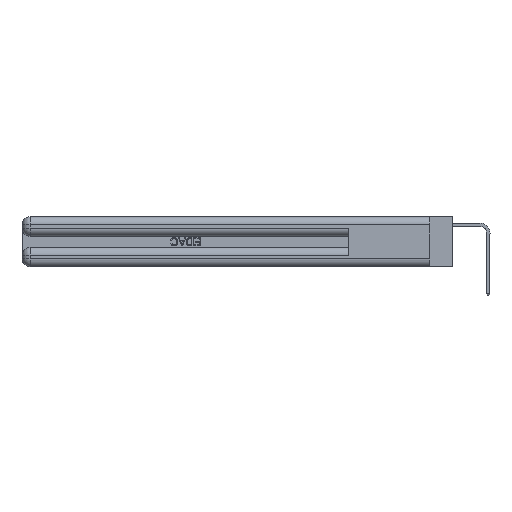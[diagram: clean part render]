
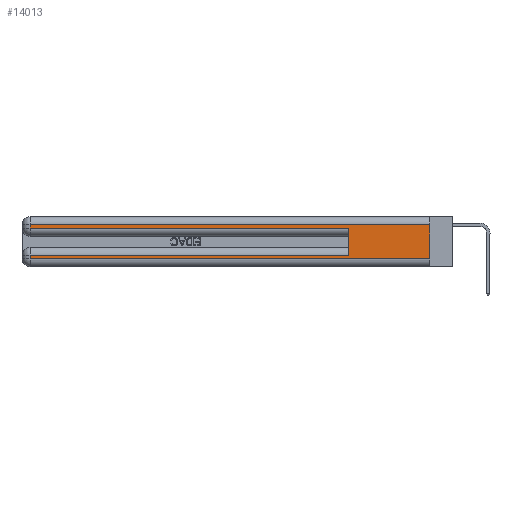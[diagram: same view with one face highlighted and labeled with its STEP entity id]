
A CAD part, left-side view. The second image highlights one B-rep face of the part: STEP entity #14013.
In plain terms, the highlighted planar face has unit normal (-1, 0, 0).
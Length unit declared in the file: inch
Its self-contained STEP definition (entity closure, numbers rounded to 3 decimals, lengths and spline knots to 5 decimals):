
#385 = VERTEX_POINT ( 'NONE', #19764 ) ;
#871 = EDGE_LOOP ( 'NONE', ( #8453, #5865, #25730, #26831, #24875, #24241, #18134, #9044 ) ) ;
#1074 = VERTEX_POINT ( 'NONE', #26707 ) ;
#1160 = VECTOR ( 'NONE', #17852, 39.37008 ) ;
#1462 = EDGE_CURVE ( 'NONE', #13988, #29570, #9830, .T. ) ;
#2735 = CARTESIAN_POINT ( 'NONE',  ( 0., 0.6, 0.145 ) ) ;
#3069 = VERTEX_POINT ( 'NONE', #13011 ) ;
#3277 = LINE ( 'NONE', #25673, #24214 ) ;
#4062 = CARTESIAN_POINT ( 'NONE',  ( 0., 2.94, 0.37 ) ) ;
#4281 = VERTEX_POINT ( 'NONE', #10620 ) ;
#5865 = ORIENTED_EDGE ( 'NONE', *, *, #6195, .T. ) ;
#6195 = EDGE_CURVE ( 'NONE', #385, #13988, #25769, .T. ) ;
#6279 = PLANE ( 'NONE',  #23796 ) ;
#7234 = DIRECTION ( 'NONE',  ( 0., 1., 0. ) ) ;
#7324 = DIRECTION ( 'NONE',  ( 0., 0., -1. ) ) ;
#7398 = LINE ( 'NONE', #4062, #1160 ) ;
#7439 = DIRECTION ( 'NONE',  ( 0., 0., 1. ) ) ;
#8453 = ORIENTED_EDGE ( 'NONE', *, *, #9283, .F. ) ;
#8616 = DIRECTION ( 'NONE',  ( 1., 0., 0. ) ) ;
#9044 = ORIENTED_EDGE ( 'NONE', *, *, #14496, .T. ) ;
#9283 = EDGE_CURVE ( 'NONE', #385, #25598, #14305, .T. ) ;
#9304 = LINE ( 'NONE', #13502, #20810 ) ;
#9428 = VECTOR ( 'NONE', #21747, 39.37008 ) ;
#9830 = LINE ( 'NONE', #23413, #22073 ) ;
#10157 = CARTESIAN_POINT ( 'NONE',  ( 0., 0., 0.31 ) ) ;
#10620 = CARTESIAN_POINT ( 'NONE',  ( 0., 2.94, 0.06 ) ) ;
#12469 = DIRECTION ( 'NONE',  ( 0., 1., 0. ) ) ;
#13011 = CARTESIAN_POINT ( 'NONE',  ( 0., 0.6, 0.285 ) ) ;
#13502 = CARTESIAN_POINT ( 'NONE',  ( 0., 0., 0.285 ) ) ;
#13506 = VECTOR ( 'NONE', #12469, 39.37008 ) ;
#13988 = VERTEX_POINT ( 'NONE', #22283 ) ;
#14013 = ADVANCED_FACE ( 'NONE', ( #28584 ), #6279, .F. ) ;
#14305 = LINE ( 'NONE', #24133, #25836 ) ;
#14496 = EDGE_CURVE ( 'NONE', #4281, #25598, #27802, .T. ) ;
#14603 = CARTESIAN_POINT ( 'NONE',  ( 0., 0.6, 0.085 ) ) ;
#14954 = VERTEX_POINT ( 'NONE', #14603 ) ;
#14994 = DIRECTION ( 'NONE',  ( 0., 0., -1. ) ) ;
#15809 = DIRECTION ( 'NONE',  ( 0., -1., 0. ) ) ;
#17852 = DIRECTION ( 'NONE',  ( 0., 0., -1. ) ) ;
#18134 = ORIENTED_EDGE ( 'NONE', *, *, #19094, .T. ) ;
#18166 = CARTESIAN_POINT ( 'NONE',  ( 0., 0., 0.06 ) ) ;
#19094 = EDGE_CURVE ( 'NONE', #1074, #4281, #7398, .T. ) ;
#19764 = CARTESIAN_POINT ( 'NONE',  ( 0., 0., 0.31 ) ) ;
#20550 = VECTOR ( 'NONE', #7439, 39.37008 ) ;
#20640 = EDGE_CURVE ( 'NONE', #14954, #1074, #3277, .T. ) ;
#20810 = VECTOR ( 'NONE', #15809, 39.37008 ) ;
#21747 = DIRECTION ( 'NONE',  ( 0., -1., 0. ) ) ;
#22073 = VECTOR ( 'NONE', #7324, 39.37008 ) ;
#22283 = CARTESIAN_POINT ( 'NONE',  ( 0., 2.94, 0.31 ) ) ;
#22383 = CARTESIAN_POINT ( 'NONE',  ( 0., 0., 0.37 ) ) ;
#23413 = CARTESIAN_POINT ( 'NONE',  ( 0., 2.94, 0.37 ) ) ;
#23796 = AXIS2_PLACEMENT_3D ( 'NONE', #22383, #8616, #24698 ) ;
#23970 = CARTESIAN_POINT ( 'NONE',  ( 0., 0., 0.06 ) ) ;
#24133 = CARTESIAN_POINT ( 'NONE',  ( 0., 0., 0.37 ) ) ;
#24214 = VECTOR ( 'NONE', #7234, 39.37008 ) ;
#24241 = ORIENTED_EDGE ( 'NONE', *, *, #20640, .T. ) ;
#24698 = DIRECTION ( 'NONE',  ( 0., 0., -1. ) ) ;
#24875 = ORIENTED_EDGE ( 'NONE', *, *, #28400, .F. ) ;
#25598 = VERTEX_POINT ( 'NONE', #18166 ) ;
#25673 = CARTESIAN_POINT ( 'NONE',  ( 0., 0., 0.085 ) ) ;
#25730 = ORIENTED_EDGE ( 'NONE', *, *, #1462, .T. ) ;
#25769 = LINE ( 'NONE', #10157, #13506 ) ;
#25836 = VECTOR ( 'NONE', #14994, 39.37008 ) ;
#26707 = CARTESIAN_POINT ( 'NONE',  ( 0., 2.94, 0.085 ) ) ;
#26831 = ORIENTED_EDGE ( 'NONE', *, *, #29935, .T. ) ;
#27802 = LINE ( 'NONE', #23970, #9428 ) ;
#27910 = CARTESIAN_POINT ( 'NONE',  ( 0., 2.94, 0.285 ) ) ;
#28140 = LINE ( 'NONE', #2735, #20550 ) ;
#28400 = EDGE_CURVE ( 'NONE', #14954, #3069, #28140, .T. ) ;
#28584 = FACE_OUTER_BOUND ( 'NONE', #871, .T. ) ;
#29570 = VERTEX_POINT ( 'NONE', #27910 ) ;
#29935 = EDGE_CURVE ( 'NONE', #29570, #3069, #9304, .T. ) ;
